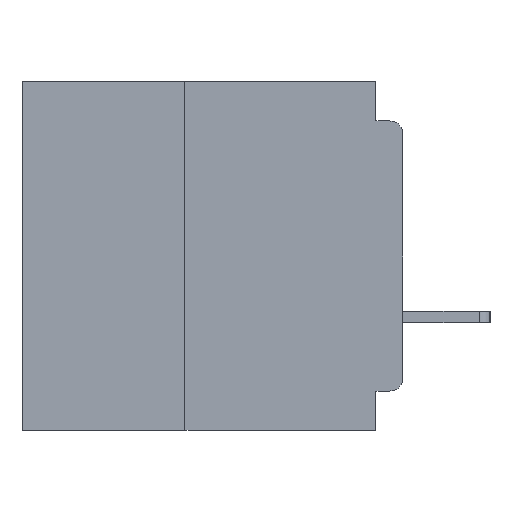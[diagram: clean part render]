
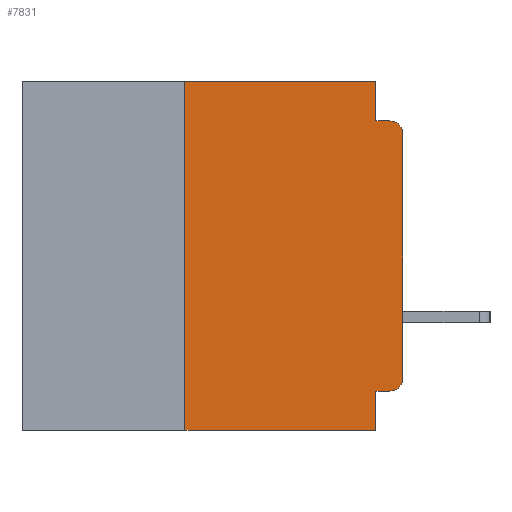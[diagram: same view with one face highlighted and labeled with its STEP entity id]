
A CAD part, left-side view. The second image highlights one B-rep face of the part: STEP entity #7831.
In plain terms, the highlighted planar face has unit normal (-1, 0, 0).
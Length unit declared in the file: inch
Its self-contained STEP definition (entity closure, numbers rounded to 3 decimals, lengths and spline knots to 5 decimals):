
#54 = EDGE_CURVE ( 'NONE', #3593, #32740, #1543, .T. ) ;
#233 = EDGE_CURVE ( 'NONE', #18791, #54327, #4487, .T. ) ;
#1543 = CIRCLE ( 'NONE', #45877, 0.015 ) ;
#2942 = DIRECTION ( 'NONE',  ( 0., 0., -1. ) ) ;
#3593 = VERTEX_POINT ( 'NONE', #7479 ) ;
#3835 = ORIENTED_EDGE ( 'NONE', *, *, #45816, .F. ) ;
#4487 = LINE ( 'NONE', #24636, #51445 ) ;
#4526 = CARTESIAN_POINT ( 'NONE',  ( 0., 0.015, -0.34 ) ) ;
#5204 = CARTESIAN_POINT ( 'NONE',  ( 0., 0.015, -0.06 ) ) ;
#6316 = CARTESIAN_POINT ( 'NONE',  ( 0., 0.437, 0. ) ) ;
#7479 = CARTESIAN_POINT ( 'NONE',  ( 0., 0., -0.06 ) ) ;
#7831 = ADVANCED_FACE ( 'NONE', ( #20713 ), #15077, .F. ) ;
#9128 = DIRECTION ( 'NONE',  ( 0., 0., -1. ) ) ;
#9801 = DIRECTION ( 'NONE',  ( 0., 0., -1. ) ) ;
#10531 = LINE ( 'NONE', #39290, #57497 ) ;
#10892 = DIRECTION ( 'NONE',  ( 0., 0., -1. ) ) ;
#11529 = CARTESIAN_POINT ( 'NONE',  ( 0., 0.437, 0. ) ) ;
#12155 = ORIENTED_EDGE ( 'NONE', *, *, #17613, .T. ) ;
#12246 = EDGE_CURVE ( 'NONE', #54172, #19285, #10531, .T. ) ;
#12623 = CARTESIAN_POINT ( 'NONE',  ( 0., 0.015, -0.355 ) ) ;
#13458 = CARTESIAN_POINT ( 'NONE',  ( 0., 0.031, -0.355 ) ) ;
#14505 = ORIENTED_EDGE ( 'NONE', *, *, #49847, .F. ) ;
#14939 = VERTEX_POINT ( 'NONE', #12623 ) ;
#15077 = PLANE ( 'NONE',  #44359 ) ;
#15904 = ORIENTED_EDGE ( 'NONE', *, *, #55964, .F. ) ;
#16151 = DIRECTION ( 'NONE',  ( 0., -1., 0. ) ) ;
#17251 = EDGE_CURVE ( 'NONE', #18356, #27591, #33714, .T. ) ;
#17613 = EDGE_CURVE ( 'NONE', #14939, #31374, #37948, .T. ) ;
#18356 = VERTEX_POINT ( 'NONE', #34665 ) ;
#18791 = VERTEX_POINT ( 'NONE', #56953 ) ;
#18863 = AXIS2_PLACEMENT_3D ( 'NONE', #4526, #36489, #9128 ) ;
#19019 = DIRECTION ( 'NONE',  ( 0., -1., 0. ) ) ;
#19285 = VERTEX_POINT ( 'NONE', #51311 ) ;
#20216 = DIRECTION ( 'NONE',  ( 0., 0., -1. ) ) ;
#20713 = FACE_OUTER_BOUND ( 'NONE', #29295, .T. ) ;
#22749 = CARTESIAN_POINT ( 'NONE',  ( 0., 0., -0.34 ) ) ;
#23778 = VECTOR ( 'NONE', #42374, 39.37008 ) ;
#24444 = LINE ( 'NONE', #37685, #29380 ) ;
#24636 = CARTESIAN_POINT ( 'NONE',  ( 0., 0.031, 0. ) ) ;
#25356 = CARTESIAN_POINT ( 'NONE',  ( 0., 0., 0. ) ) ;
#27591 = VERTEX_POINT ( 'NONE', #42881 ) ;
#28881 = CARTESIAN_POINT ( 'NONE',  ( 0., 0., -0.045 ) ) ;
#29295 = EDGE_LOOP ( 'NONE', ( #58693, #36560, #15904, #45598, #14505, #45686, #42411, #35766, #3835, #12155 ) ) ;
#29380 = VECTOR ( 'NONE', #50877, 39.37008 ) ;
#31153 = EDGE_CURVE ( 'NONE', #31374, #3593, #57652, .T. ) ;
#31374 = VERTEX_POINT ( 'NONE', #22749 ) ;
#31806 = LINE ( 'NONE', #11529, #54438 ) ;
#32740 = VERTEX_POINT ( 'NONE', #37810 ) ;
#33714 = LINE ( 'NONE', #56268, #44360 ) ;
#34665 = CARTESIAN_POINT ( 'NONE',  ( 0., 0.25, -0.4 ) ) ;
#34946 = VECTOR ( 'NONE', #19019, 39.37008 ) ;
#35766 = ORIENTED_EDGE ( 'NONE', *, *, #12246, .F. ) ;
#36489 = DIRECTION ( 'NONE',  ( -1., 0., 0. ) ) ;
#36560 = ORIENTED_EDGE ( 'NONE', *, *, #54, .T. ) ;
#37163 = DIRECTION ( 'NONE',  ( -1., 0., 0. ) ) ;
#37685 = CARTESIAN_POINT ( 'NONE',  ( 0., 0., -0.355 ) ) ;
#37810 = CARTESIAN_POINT ( 'NONE',  ( 0., 0.015, -0.045 ) ) ;
#37948 = CIRCLE ( 'NONE', #18863, 0.015 ) ;
#38244 = DIRECTION ( 'NONE',  ( 1., 0., 0. ) ) ;
#39290 = CARTESIAN_POINT ( 'NONE',  ( 0., 0.031, -0.4 ) ) ;
#42269 = EDGE_CURVE ( 'NONE', #18356, #19285, #45548, .T. ) ;
#42374 = DIRECTION ( 'NONE',  ( 0., -1., 0. ) ) ;
#42411 = ORIENTED_EDGE ( 'NONE', *, *, #42269, .T. ) ;
#42852 = DIRECTION ( 'NONE',  ( 0., 0., 1. ) ) ;
#42881 = CARTESIAN_POINT ( 'NONE',  ( 0., 0.25, 0. ) ) ;
#43595 = DIRECTION ( 'NONE',  ( 0., 0., 1. ) ) ;
#44210 = VECTOR ( 'NONE', #43595, 39.37008 ) ;
#44359 = AXIS2_PLACEMENT_3D ( 'NONE', #6316, #38244, #10892 ) ;
#44360 = VECTOR ( 'NONE', #42852, 39.37008 ) ;
#45036 = LINE ( 'NONE', #28881, #23778 ) ;
#45548 = LINE ( 'NONE', #46188, #34946 ) ;
#45598 = ORIENTED_EDGE ( 'NONE', *, *, #233, .F. ) ;
#45686 = ORIENTED_EDGE ( 'NONE', *, *, #17251, .F. ) ;
#45816 = EDGE_CURVE ( 'NONE', #14939, #54172, #24444, .T. ) ;
#45877 = AXIS2_PLACEMENT_3D ( 'NONE', #5204, #37163, #9801 ) ;
#46188 = CARTESIAN_POINT ( 'NONE',  ( 0., 0.437, -0.4 ) ) ;
#49847 = EDGE_CURVE ( 'NONE', #27591, #18791, #31806, .T. ) ;
#50779 = CARTESIAN_POINT ( 'NONE',  ( 0., 0.031, -0.045 ) ) ;
#50877 = DIRECTION ( 'NONE',  ( 0., 1., 0. ) ) ;
#51311 = CARTESIAN_POINT ( 'NONE',  ( 0., 0.031, -0.4 ) ) ;
#51445 = VECTOR ( 'NONE', #20216, 39.37008 ) ;
#54172 = VERTEX_POINT ( 'NONE', #13458 ) ;
#54327 = VERTEX_POINT ( 'NONE', #50779 ) ;
#54438 = VECTOR ( 'NONE', #16151, 39.37008 ) ;
#55964 = EDGE_CURVE ( 'NONE', #54327, #32740, #45036, .T. ) ;
#56268 = CARTESIAN_POINT ( 'NONE',  ( 0., 0.25, -0.4 ) ) ;
#56953 = CARTESIAN_POINT ( 'NONE',  ( 0., 0.031, 0. ) ) ;
#57497 = VECTOR ( 'NONE', #2942, 39.37008 ) ;
#57652 = LINE ( 'NONE', #25356, #44210 ) ;
#58693 = ORIENTED_EDGE ( 'NONE', *, *, #31153, .T. ) ;
